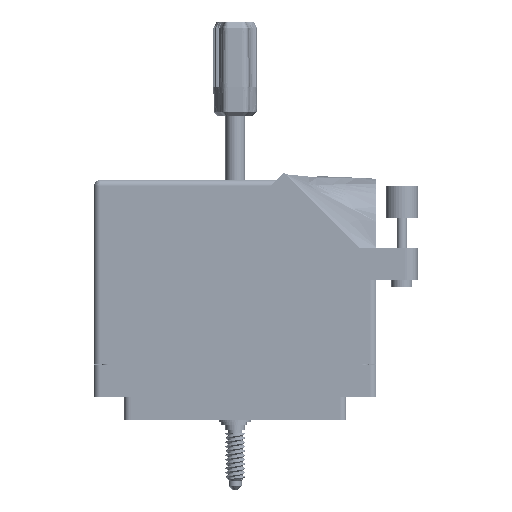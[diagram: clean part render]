
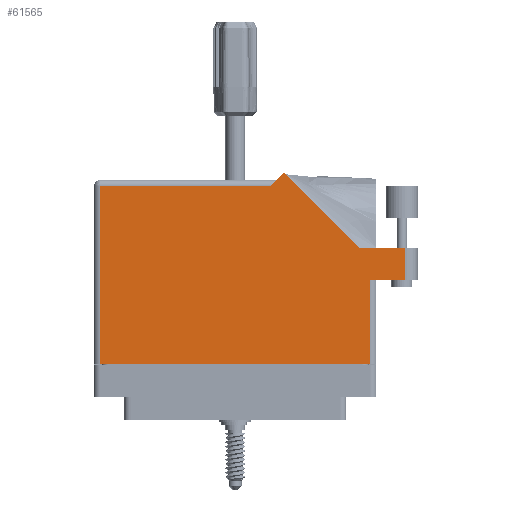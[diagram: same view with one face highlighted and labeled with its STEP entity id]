
A CAD part, front view. The second image highlights one B-rep face of the part: STEP entity #61565.
In plain terms, the highlighted face is planar.
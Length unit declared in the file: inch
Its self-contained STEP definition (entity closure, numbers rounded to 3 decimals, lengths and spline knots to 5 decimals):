
#40 = VECTOR ( 'NONE', #44172, 39.37008 ) ;
#543 = VERTEX_POINT ( 'NONE', #71407 ) ;
#2270 = CARTESIAN_POINT ( 'NONE',  ( -1.297, -0.1, 0.617 ) ) ;
#2846 = DIRECTION ( 'NONE',  ( 1., 0., 0. ) ) ;
#4008 = VERTEX_POINT ( 'NONE', #4606 ) ;
#4606 = CARTESIAN_POINT ( 'NONE',  ( 1.634, 1.022, 0.617 ) ) ;
#5375 = VECTOR ( 'NONE', #52926, 39.37008 ) ;
#6166 = DIRECTION ( 'NONE',  ( 1., 0., 0. ) ) ;
#7123 = CARTESIAN_POINT ( 'NONE',  ( -1.359, 1.675, 0.617 ) ) ;
#7439 = EDGE_CURVE ( 'NONE', #4008, #79865, #20894, .T. ) ;
#7777 = LINE ( 'NONE', #52592, #82207 ) ;
#8361 = AXIS2_PLACEMENT_3D ( 'NONE', #7123, #60497, #20016 ) ;
#9177 = CARTESIAN_POINT ( 'NONE',  ( -1.297, 1.613, 0.617 ) ) ;
#10332 = CARTESIAN_POINT ( 'NONE',  ( 0.46971, 1.74571, 0.617 ) ) ;
#11571 = LINE ( 'NONE', #37104, #54542 ) ;
#12374 = EDGE_CURVE ( 'NONE', #52934, #13594, #23211, .T. ) ;
#12952 = ORIENTED_EDGE ( 'NONE', *, *, #12374, .T. ) ;
#13560 = PLANE ( 'NONE',  #8361 ) ;
#13594 = VERTEX_POINT ( 'NONE', #70579 ) ;
#18793 = CARTESIAN_POINT ( 'NONE',  ( 1.359, 0.715, 0.617 ) ) ;
#20016 = DIRECTION ( 'NONE',  ( -1., 0., 0. ) ) ;
#20894 = LINE ( 'NONE', #75571, #35736 ) ;
#23211 = LINE ( 'NONE', #18793, #49430 ) ;
#24338 = ORIENTED_EDGE ( 'NONE', *, *, #80011, .T. ) ;
#25217 = LINE ( 'NONE', #2270, #40 ) ;
#30788 = LINE ( 'NONE', #76705, #57060 ) ;
#33398 = FACE_OUTER_BOUND ( 'NONE', #40164, .T. ) ;
#35441 = EDGE_CURVE ( 'NONE', #52423, #543, #30788, .T. ) ;
#35736 = VECTOR ( 'NONE', #82298, 39.37008 ) ;
#37104 = CARTESIAN_POINT ( 'NONE',  ( 1.634, 1.022, 0.617 ) ) ;
#37692 = DIRECTION ( 'NONE',  ( 0., 1., 0. ) ) ;
#39397 = DIRECTION ( 'NONE',  ( -1., 0., 0. ) ) ;
#39976 = ORIENTED_EDGE ( 'NONE', *, *, #53641, .T. ) ;
#40164 = EDGE_LOOP ( 'NONE', ( #12952, #76859, #85158, #71814, #39976, #24338, #59183, #72759, #76494 ) ) ;
#40691 = CARTESIAN_POINT ( 'NONE',  ( 0.337, 1.613, 0.617 ) ) ;
#42525 = VERTEX_POINT ( 'NONE', #10332 ) ;
#43351 = VERTEX_POINT ( 'NONE', #9177 ) ;
#44172 = DIRECTION ( 'NONE',  ( 0., -1., 0. ) ) ;
#46368 = LINE ( 'NONE', #79573, #5375 ) ;
#49430 = VECTOR ( 'NONE', #6166, 39.37008 ) ;
#49703 = CARTESIAN_POINT ( 'NONE',  ( 1.19342, 1.022, 0.617 ) ) ;
#52423 = VERTEX_POINT ( 'NONE', #68765 ) ;
#52592 = CARTESIAN_POINT ( 'NONE',  ( -1.359, 1.613, 0.617 ) ) ;
#52926 = DIRECTION ( 'NONE',  ( -0.707, -0.707, 0. ) ) ;
#52934 = VERTEX_POINT ( 'NONE', #66643 ) ;
#53641 = EDGE_CURVE ( 'NONE', #42525, #70316, #46368, .T. ) ;
#54542 = VECTOR ( 'NONE', #37692, 39.37008 ) ;
#57060 = VECTOR ( 'NONE', #2846, 39.37008 ) ;
#59183 = ORIENTED_EDGE ( 'NONE', *, *, #68428, .T. ) ;
#60497 = DIRECTION ( 'NONE',  ( 0., 0., -1. ) ) ;
#60503 = EDGE_CURVE ( 'NONE', #13594, #4008, #11571, .T. ) ;
#61345 = EDGE_CURVE ( 'NONE', #543, #52934, #65977, .T. ) ;
#61565 = ADVANCED_FACE ( 'NONE', ( #33398 ), #13560, .F. ) ;
#61762 = VECTOR ( 'NONE', #82769, 39.37008 ) ;
#63779 = DIRECTION ( 'NONE',  ( -0.707, 0.707, 0. ) ) ;
#64498 = VECTOR ( 'NONE', #63779, 39.37008 ) ;
#65736 = CARTESIAN_POINT ( 'NONE',  ( 1.19342, 1.022, 0.617 ) ) ;
#65977 = LINE ( 'NONE', #76905, #61762 ) ;
#66643 = CARTESIAN_POINT ( 'NONE',  ( 1.297, 0.715, 0.617 ) ) ;
#68428 = EDGE_CURVE ( 'NONE', #43351, #52423, #25217, .T. ) ;
#68765 = CARTESIAN_POINT ( 'NONE',  ( -1.297, -0.1, 0.617 ) ) ;
#70316 = VERTEX_POINT ( 'NONE', #40691 ) ;
#70579 = CARTESIAN_POINT ( 'NONE',  ( 1.634, 0.715, 0.617 ) ) ;
#71407 = CARTESIAN_POINT ( 'NONE',  ( 1.297, -0.1, 0.617 ) ) ;
#71814 = ORIENTED_EDGE ( 'NONE', *, *, #78865, .T. ) ;
#72759 = ORIENTED_EDGE ( 'NONE', *, *, #35441, .T. ) ;
#75571 = CARTESIAN_POINT ( 'NONE',  ( 1.759, 1.022, 0.617 ) ) ;
#75965 = LINE ( 'NONE', #49703, #64498 ) ;
#76494 = ORIENTED_EDGE ( 'NONE', *, *, #61345, .T. ) ;
#76705 = CARTESIAN_POINT ( 'NONE',  ( -1.359, -0.1, 0.617 ) ) ;
#76859 = ORIENTED_EDGE ( 'NONE', *, *, #60503, .T. ) ;
#76905 = CARTESIAN_POINT ( 'NONE',  ( 1.297, 0.715, 0.617 ) ) ;
#78865 = EDGE_CURVE ( 'NONE', #79865, #42525, #75965, .T. ) ;
#79573 = CARTESIAN_POINT ( 'NONE',  ( 0.399, 1.675, 0.617 ) ) ;
#79865 = VERTEX_POINT ( 'NONE', #65736 ) ;
#80011 = EDGE_CURVE ( 'NONE', #70316, #43351, #7777, .T. ) ;
#82207 = VECTOR ( 'NONE', #39397, 39.37008 ) ;
#82298 = DIRECTION ( 'NONE',  ( -1., 0., 0. ) ) ;
#82769 = DIRECTION ( 'NONE',  ( 0., 1., 0. ) ) ;
#85158 = ORIENTED_EDGE ( 'NONE', *, *, #7439, .T. ) ;
